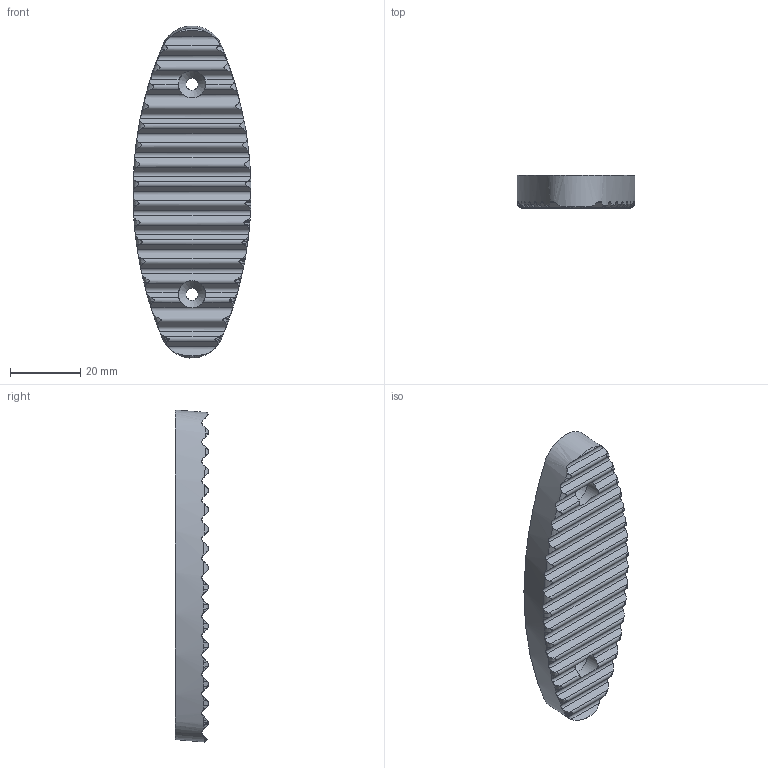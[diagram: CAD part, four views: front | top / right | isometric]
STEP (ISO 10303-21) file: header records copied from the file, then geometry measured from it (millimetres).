
FILE_DESCRIPTION(/* description */ (''),/* implementation_level */ '2;1');
FILE_NAME(/* name */ 'Mares Leg Cover.step',/* time_stamp */ '2022-04-14T02:27:06-04:00',/* author */ (''),/* organization */ (''),/* preprocessor_version */ 'ST-DEVELOPER v18.1',/* originating_system */ 'Autodesk Translation Framework v10.14.0.1471',/* authorisation */ '');
FILE_SCHEMA (('AUTOMOTIVE_DESIGN { 1 0 10303 214 3 1 1 }'));
Length unit declared in the file: millimetre
Products named in the file (1): Mares Leg Cover
Bounding box: 33.7 x 9.49 x 94.83 mm (x, y, z)
Volume: 19318.3 mm3; surface area: 7530.3 mm2
Topology: 1 solids, 1 shells, 206 faces, 612 edges, 407 vertices
Faces by surface type: bspline 113, plane 48, cylinder 41, torus 2, cone 2
Full cylindrical faces by diameter (mm): 3.505 x2, 7.798 x2
Entity records: 13586 total; most frequent: CARTESIAN_POINT 9176, ORIENTED_EDGE 1224, EDGE_CURVE 612, B_SPLINE_CURVE_WITH_KNOTS 444, DIRECTION 419, VERTEX_POINT 407, EDGE_LOOP 209, FACE_OUTER_BOUND 206
